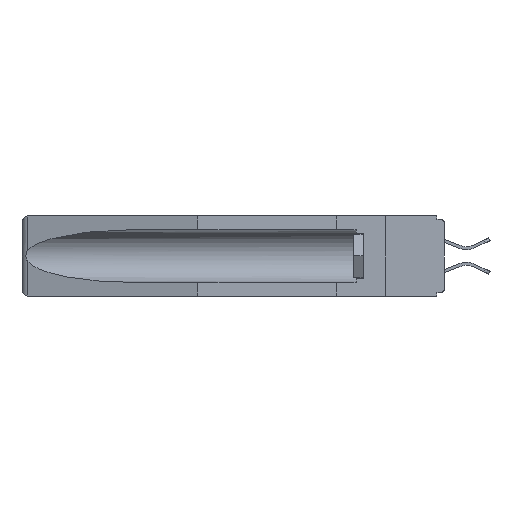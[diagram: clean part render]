
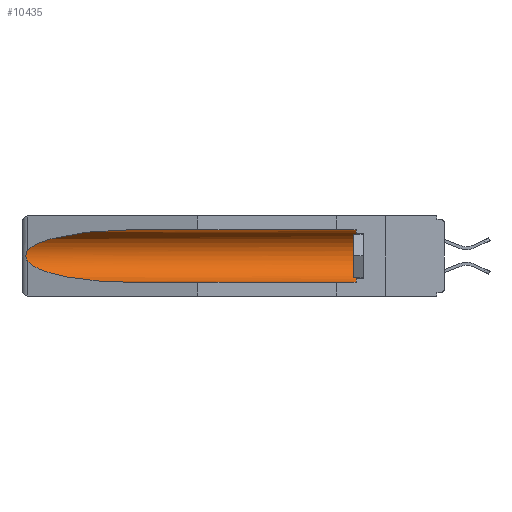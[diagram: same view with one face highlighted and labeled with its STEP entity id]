
A CAD part, left-side view. The second image highlights one B-rep face of the part: STEP entity #10435.
In plain terms, the highlighted cylindrical face has radius 2.857 mm (diameter 5.715 mm), a partial arc.
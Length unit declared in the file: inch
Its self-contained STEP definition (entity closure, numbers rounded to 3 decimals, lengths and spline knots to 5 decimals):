
#7 = VERTEX_POINT ( 'NONE', #10556 ) ;
#144 = CARTESIAN_POINT ( 'NONE',  ( 0.26537, 1.52718, -0.19328 ) ) ;
#1277 = FACE_OUTER_BOUND ( 'NONE', #14944, .T. ) ;
#1982 = VECTOR ( 'NONE', #5937, 39.37008 ) ;
#2062 = VERTEX_POINT ( 'NONE', #19587 ) ;
#2116 = DIRECTION ( 'NONE',  ( 0., 1., 0. ) ) ;
#2406 = ORIENTED_EDGE ( 'NONE', *, *, #18688, .T. ) ;
#2935 = ORIENTED_EDGE ( 'NONE', *, *, #14743, .F. ) ;
#3083 = CARTESIAN_POINT ( 'NONE',  ( 0.2675, 1.53308, -0.16763 ) ) ;
#3157 = CARTESIAN_POINT ( 'NONE',  ( 0.2673, 1.53269, -0.17917 ) ) ;
#3257 = EDGE_CURVE ( 'NONE', #2062, #20219, #13625, .T. ) ;
#3300 = CARTESIAN_POINT ( 'NONE',  ( 0.26597, 1.5296, -0.19026 ) ) ;
#3620 = B_SPLINE_CURVE_WITH_KNOTS ( 'NONE', 3,
 ( #7940, #17182, #15859, #18877, #3083, #20276, #3157, #9593, #3300, #144 ),
 .UNSPECIFIED., .F., .F.,
 ( 4, 2, 2, 2, 4 ),
 ( 0., 0.00029, 0.00058, 0.00087, 0.00117 ),
 .UNSPECIFIED. ) ;
#4147 = ORIENTED_EDGE ( 'NONE', *, *, #3257, .T. ) ;
#4515 = AXIS2_PLACEMENT_3D ( 'NONE', #19338, #13113, #12986 ) ;
#5452 = LINE ( 'NONE', #7460, #1982 ) ;
#5570 = CARTESIAN_POINT ( 'NONE',  ( 0.21114, 1.30732, -0.059 ) ) ;
#5937 = DIRECTION ( 'NONE',  ( 0., 1., 0. ) ) ;
#6063 = CARTESIAN_POINT ( 'NONE',  ( 0.155, 1.07973, -0.284 ) ) ;
#6135 = CARTESIAN_POINT ( 'NONE',  ( 0.21114, 1.30732, -0.284 ) ) ;
#6247 = ORIENTED_EDGE ( 'NONE', *, *, #17510, .T. ) ;
#6622 = DIRECTION ( 'NONE',  ( 0., 1., 0. ) ) ;
#6882 = DIRECTION ( 'NONE',  ( 0., 0., 1. ) ) ;
#7460 = CARTESIAN_POINT ( 'NONE',  ( 0.155, -0.30754, -0.284 ) ) ;
#7692 = ORIENTED_EDGE ( 'NONE', *, *, #14203, .T. ) ;
#7940 = CARTESIAN_POINT ( 'NONE',  ( 0.26537, 1.52718, -0.14972 ) ) ;
#8374 = CARTESIAN_POINT ( 'NONE',  ( 0.155, 0.126, -0.059 ) ) ;
#9254 = CARTESIAN_POINT ( 'NONE',  ( 0.26537, 1.52718, -0.19328 ) ) ;
#9593 = CARTESIAN_POINT ( 'NONE',  ( 0.26655, 1.53094, -0.18657 ) ) ;
#10435 = ADVANCED_FACE ( 'NONE', ( #1277 ), #19209, .F. ) ;
#10556 = CARTESIAN_POINT ( 'NONE',  ( 0.155, 1.07973, -0.284 ) ) ;
#10720 = VERTEX_POINT ( 'NONE', #14606 ) ;
#10951 =( BOUNDED_CURVE ( )  B_SPLINE_CURVE ( 3, ( #14975, #5570, #19674, #14848 ),
 .UNSPECIFIED., .F., .T. ) 
 B_SPLINE_CURVE_WITH_KNOTS ( ( 4, 4 ),
 ( 4.71239, 6.08839 ),
 .UNSPECIFIED. ) 
 CURVE ( )  GEOMETRIC_REPRESENTATION_ITEM ( )  RATIONAL_B_SPLINE_CURVE ( ( 1., 0.848, 0.848, 1. ) ) 
 REPRESENTATION_ITEM ( '' )  );
#11430 = EDGE_CURVE ( 'NONE', #15014, #7, #14579, .T. ) ;
#12035 = AXIS2_PLACEMENT_3D ( 'NONE', #14907, #2116, #6882 ) ;
#12445 = CARTESIAN_POINT ( 'NONE',  ( 0.155, 1.07973, -0.059 ) ) ;
#12986 = DIRECTION ( 'NONE',  ( 0., 0., 1. ) ) ;
#13113 = DIRECTION ( 'NONE',  ( 0., -1., 0. ) ) ;
#13461 = VERTEX_POINT ( 'NONE', #12445 ) ;
#13625 = CIRCLE ( 'NONE', #4515, 0.1125 ) ;
#14203 = EDGE_CURVE ( 'NONE', #20219, #13461, #15760, .T. ) ;
#14576 = CARTESIAN_POINT ( 'NONE',  ( 0.26537, 1.52718, -0.19328 ) ) ;
#14579 =( BOUNDED_CURVE ( )  B_SPLINE_CURVE ( 3, ( #9254, #17235, #6135, #6063 ),
 .UNSPECIFIED., .F., .F. ) 
 B_SPLINE_CURVE_WITH_KNOTS ( ( 4, 4 ),
 ( 0.1948, 1.5708 ),
 .UNSPECIFIED. ) 
 CURVE ( )  GEOMETRIC_REPRESENTATION_ITEM ( )  RATIONAL_B_SPLINE_CURVE ( ( 1., 0.848, 0.848, 1. ) ) 
 REPRESENTATION_ITEM ( '' )  );
#14606 = CARTESIAN_POINT ( 'NONE',  ( 0.26537, 1.52718, -0.14972 ) ) ;
#14743 = EDGE_CURVE ( 'NONE', #2062, #7, #5452, .T. ) ;
#14848 = CARTESIAN_POINT ( 'NONE',  ( 0.26537, 1.52718, -0.14972 ) ) ;
#14907 = CARTESIAN_POINT ( 'NONE',  ( 0.155, -0.30754, -0.1715 ) ) ;
#14944 = EDGE_LOOP ( 'NONE', ( #6247, #2406, #17429, #2935, #4147, #7692 ) ) ;
#14975 = CARTESIAN_POINT ( 'NONE',  ( 0.155, 1.07973, -0.059 ) ) ;
#15014 = VERTEX_POINT ( 'NONE', #14576 ) ;
#15265 = VECTOR ( 'NONE', #6622, 39.37008 ) ;
#15760 = LINE ( 'NONE', #15995, #15265 ) ;
#15859 = CARTESIAN_POINT ( 'NONE',  ( 0.26654, 1.53092, -0.15636 ) ) ;
#15995 = CARTESIAN_POINT ( 'NONE',  ( 0.155, -0.30754, -0.059 ) ) ;
#17182 = CARTESIAN_POINT ( 'NONE',  ( 0.26597, 1.52961, -0.15275 ) ) ;
#17235 = CARTESIAN_POINT ( 'NONE',  ( 0.25451, 1.48313, -0.24835 ) ) ;
#17429 = ORIENTED_EDGE ( 'NONE', *, *, #11430, .T. ) ;
#17510 = EDGE_CURVE ( 'NONE', #13461, #10720, #10951, .T. ) ;
#18688 = EDGE_CURVE ( 'NONE', #10720, #15014, #3620, .T. ) ;
#18877 = CARTESIAN_POINT ( 'NONE',  ( 0.2673, 1.5327, -0.16383 ) ) ;
#19209 = CYLINDRICAL_SURFACE ( 'NONE', #12035, 0.1125 ) ;
#19338 = CARTESIAN_POINT ( 'NONE',  ( 0.155, 0.126, -0.1715 ) ) ;
#19587 = CARTESIAN_POINT ( 'NONE',  ( 0.155, 0.126, -0.284 ) ) ;
#19674 = CARTESIAN_POINT ( 'NONE',  ( 0.25451, 1.48313, -0.09465 ) ) ;
#20219 = VERTEX_POINT ( 'NONE', #8374 ) ;
#20276 = CARTESIAN_POINT ( 'NONE',  ( 0.2675, 1.53308, -0.17534 ) ) ;
